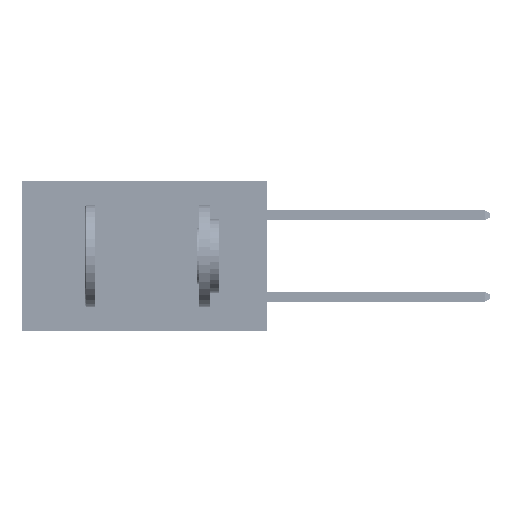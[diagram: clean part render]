
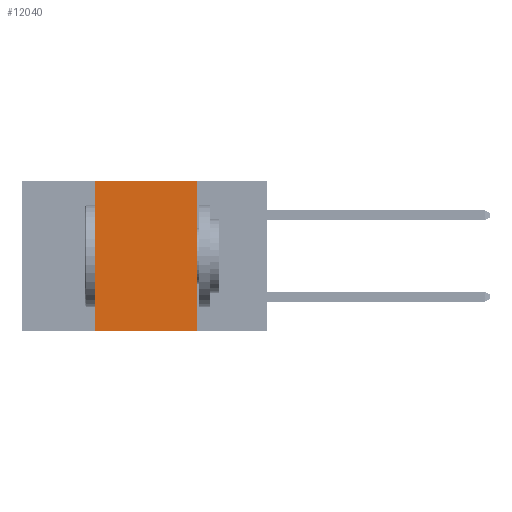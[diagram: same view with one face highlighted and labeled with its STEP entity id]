
A CAD part, left-side view. The second image highlights one B-rep face of the part: STEP entity #12040.
In plain terms, the highlighted planar face has unit normal (-1, 0, 0).
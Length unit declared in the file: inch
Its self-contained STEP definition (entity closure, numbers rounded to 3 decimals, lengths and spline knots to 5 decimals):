
#1797 = ORIENTED_EDGE ( 'NONE', *, *, #40394, .F. ) ;
#3620 = VERTEX_POINT ( 'NONE', #22036 ) ;
#5494 = EDGE_CURVE ( 'NONE', #30567, #50841, #40866, .T. ) ;
#8477 = DIRECTION ( 'NONE',  ( 0., -1., 0. ) ) ;
#9195 = EDGE_CURVE ( 'NONE', #43061, #50841, #47342, .T. ) ;
#12040 = ADVANCED_FACE ( 'NONE', ( #27828 ), #18677, .F. ) ;
#14018 = DIRECTION ( 'NONE',  ( 1., 0., 0. ) ) ;
#16929 = CARTESIAN_POINT ( 'NONE',  ( 0., 0.6, 0. ) ) ;
#18677 = PLANE ( 'NONE',  #35029 ) ;
#19900 = ORIENTED_EDGE ( 'NONE', *, *, #34413, .F. ) ;
#22036 = CARTESIAN_POINT ( 'NONE',  ( 0., 0.42, 0. ) ) ;
#24724 = CARTESIAN_POINT ( 'NONE',  ( 0., 0.17, 0. ) ) ;
#25296 = CARTESIAN_POINT ( 'NONE',  ( 0., 0.6, -0.37 ) ) ;
#26651 = VECTOR ( 'NONE', #31214, 39.37008 ) ;
#27288 = LINE ( 'NONE', #16929, #42838 ) ;
#27828 = FACE_OUTER_BOUND ( 'NONE', #37830, .T. ) ;
#30567 = VERTEX_POINT ( 'NONE', #35287 ) ;
#31214 = DIRECTION ( 'NONE',  ( 0., 0., 1. ) ) ;
#32390 = ORIENTED_EDGE ( 'NONE', *, *, #5494, .T. ) ;
#34014 = VECTOR ( 'NONE', #37666, 39.37008 ) ;
#34413 = EDGE_CURVE ( 'NONE', #3620, #43061, #27288, .T. ) ;
#34599 = CARTESIAN_POINT ( 'NONE',  ( 0., 0.17, 0. ) ) ;
#35029 = AXIS2_PLACEMENT_3D ( 'NONE', #46490, #14018, #42988 ) ;
#35287 = CARTESIAN_POINT ( 'NONE',  ( 0., 0.42, -0.37 ) ) ;
#35403 = CARTESIAN_POINT ( 'NONE',  ( 0., 0.42, 0. ) ) ;
#36788 = VECTOR ( 'NONE', #49056, 39.37008 ) ;
#37288 = CARTESIAN_POINT ( 'NONE',  ( 0., 0.17, -0.37 ) ) ;
#37666 = DIRECTION ( 'NONE',  ( 0., -1., 0. ) ) ;
#37830 = EDGE_LOOP ( 'NONE', ( #47271, #19900, #1797, #32390 ) ) ;
#40394 = EDGE_CURVE ( 'NONE', #30567, #3620, #47805, .T. ) ;
#40866 = LINE ( 'NONE', #25296, #34014 ) ;
#42838 = VECTOR ( 'NONE', #8477, 39.37008 ) ;
#42988 = DIRECTION ( 'NONE',  ( 0., 0., -1. ) ) ;
#43061 = VERTEX_POINT ( 'NONE', #34599 ) ;
#46490 = CARTESIAN_POINT ( 'NONE',  ( 0., 0.6, 0. ) ) ;
#47271 = ORIENTED_EDGE ( 'NONE', *, *, #9195, .F. ) ;
#47342 = LINE ( 'NONE', #24724, #36788 ) ;
#47805 = LINE ( 'NONE', #35403, #26651 ) ;
#49056 = DIRECTION ( 'NONE',  ( 0., 0., -1. ) ) ;
#50841 = VERTEX_POINT ( 'NONE', #37288 ) ;
